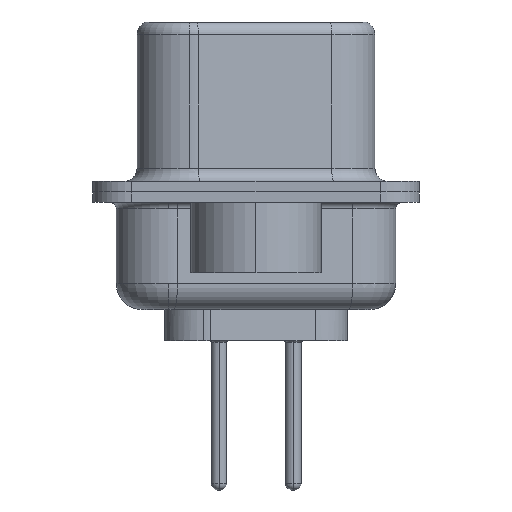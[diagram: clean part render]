
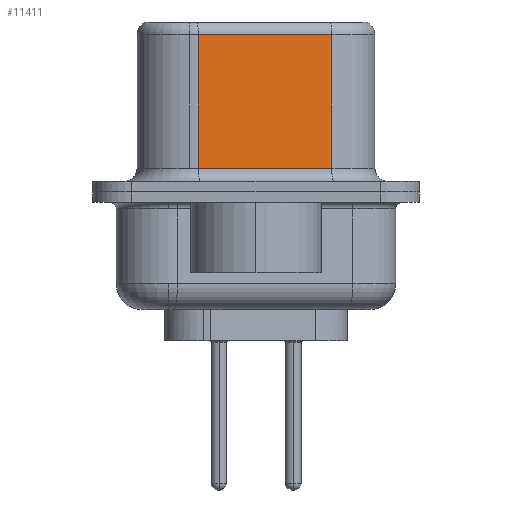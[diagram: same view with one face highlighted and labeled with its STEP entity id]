
A CAD part, left-side view. The second image highlights one B-rep face of the part: STEP entity #11411.
In plain terms, the highlighted planar face has unit normal (-0.985, -0.174, 0).
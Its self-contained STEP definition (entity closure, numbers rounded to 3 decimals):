
#382 = EDGE_CURVE ( 'NONE', #9134, #1065, #2618, .T. ) ;
#507 = EDGE_CURVE ( 'NONE', #9134, #7195, #9131, .T. ) ;
#833 = PLANE ( 'NONE',  #3947 ) ;
#1065 = VERTEX_POINT ( 'NONE', #12160 ) ;
#1378 = VERTEX_POINT ( 'NONE', #5294 ) ;
#2035 = DIRECTION ( 'NONE',  ( -0.174, 0.985, 0. ) ) ;
#2411 = ORIENTED_EDGE ( 'NONE', *, *, #507, .F. ) ;
#2618 = LINE ( 'NONE', #16719, #3834 ) ;
#3321 = CARTESIAN_POINT ( 'NONE',  ( 4.555, -2.897, 6.52 ) ) ;
#3369 = VECTOR ( 'NONE', #16083, 1000. ) ;
#3834 = VECTOR ( 'NONE', #5181, 1000. ) ;
#3943 = ORIENTED_EDGE ( 'NONE', *, *, #8312, .T. ) ;
#3947 = AXIS2_PLACEMENT_3D ( 'NONE', #3321, #7098, #2035 ) ;
#4261 = CARTESIAN_POINT ( 'NONE',  ( 4.555, -2.897, 0.9 ) ) ;
#4304 = LINE ( 'NONE', #13612, #3369 ) ;
#4806 = VECTOR ( 'NONE', #16086, 1000. ) ;
#5181 = DIRECTION ( 'NONE',  ( -0.174, 0.985, 0. ) ) ;
#5294 = CARTESIAN_POINT ( 'NONE',  ( 3.655, 2.203, 0.9 ) ) ;
#6045 = ORIENTED_EDGE ( 'NONE', *, *, #13434, .T. ) ;
#7098 = DIRECTION ( 'NONE',  ( 0.985, 0.174, 0. ) ) ;
#7195 = VERTEX_POINT ( 'NONE', #4261 ) ;
#8312 = EDGE_CURVE ( 'NONE', #1378, #7195, #4304, .T. ) ;
#9131 = LINE ( 'NONE', #14982, #10424 ) ;
#9134 = VERTEX_POINT ( 'NONE', #11091 ) ;
#9705 = DIRECTION ( 'NONE',  ( 0., 0., -1. ) ) ;
#10424 = VECTOR ( 'NONE', #9705, 1000. ) ;
#11091 = CARTESIAN_POINT ( 'NONE',  ( 4.555, -2.897, 6.02 ) ) ;
#11411 = ADVANCED_FACE ( 'NONE', ( #12478 ), #833, .F. ) ;
#11678 = EDGE_LOOP ( 'NONE', ( #2411, #12167, #6045, #3943 ) ) ;
#12160 = CARTESIAN_POINT ( 'NONE',  ( 3.655, 2.203, 6.02 ) ) ;
#12167 = ORIENTED_EDGE ( 'NONE', *, *, #382, .T. ) ;
#12478 = FACE_OUTER_BOUND ( 'NONE', #11678, .T. ) ;
#13434 = EDGE_CURVE ( 'NONE', #1065, #1378, #16342, .T. ) ;
#13533 = CARTESIAN_POINT ( 'NONE',  ( 3.655, 2.203, 6.52 ) ) ;
#13612 = CARTESIAN_POINT ( 'NONE',  ( 4.555, -2.897, 0.9 ) ) ;
#14982 = CARTESIAN_POINT ( 'NONE',  ( 4.555, -2.897, 6.52 ) ) ;
#16083 = DIRECTION ( 'NONE',  ( 0.174, -0.985, 0. ) ) ;
#16086 = DIRECTION ( 'NONE',  ( 0., 0., -1. ) ) ;
#16342 = LINE ( 'NONE', #13533, #4806 ) ;
#16719 = CARTESIAN_POINT ( 'NONE',  ( 4.555, -2.897, 6.02 ) ) ;
